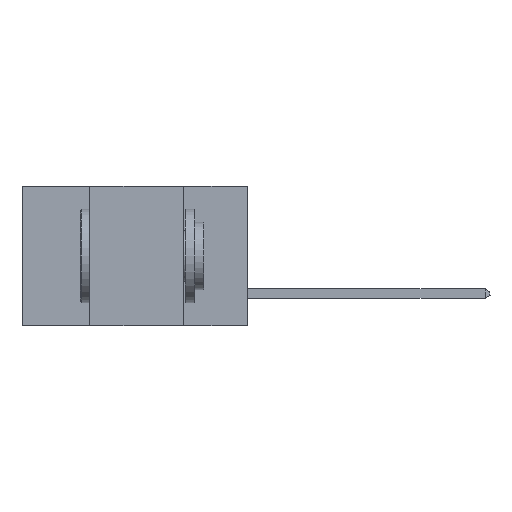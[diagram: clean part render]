
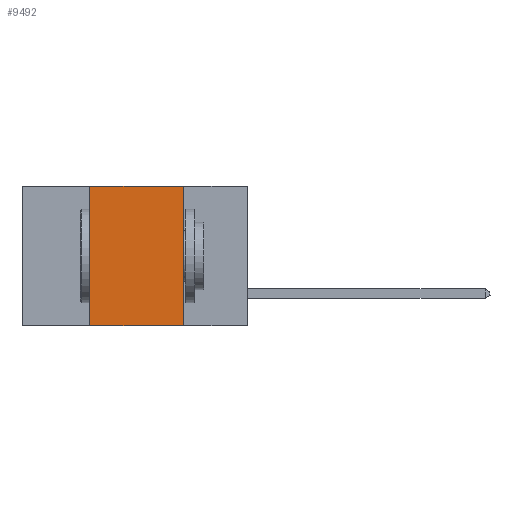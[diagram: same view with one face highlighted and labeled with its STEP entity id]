
A CAD part, left-side view. The second image highlights one B-rep face of the part: STEP entity #9492.
In plain terms, the highlighted planar face has unit normal (-1, 0, 0).
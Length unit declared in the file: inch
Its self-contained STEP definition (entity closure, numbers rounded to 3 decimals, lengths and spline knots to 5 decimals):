
#25 = AXIS2_PLACEMENT_3D ( 'NONE', #9663, #7342, #1075 ) ;
#957 = CARTESIAN_POINT ( 'NONE',  ( 0., 0.17, 0. ) ) ;
#1024 = DIRECTION ( 'NONE',  ( 0., 0., 1. ) ) ;
#1075 = DIRECTION ( 'NONE',  ( 0., 0., -1. ) ) ;
#1392 = ORIENTED_EDGE ( 'NONE', *, *, #3234, .F. ) ;
#1504 = CARTESIAN_POINT ( 'NONE',  ( 0., 0.17, 0. ) ) ;
#1588 = EDGE_CURVE ( 'NONE', #4769, #3531, #7890, .T. ) ;
#1631 = VECTOR ( 'NONE', #1024, 39.37008 ) ;
#1837 = EDGE_CURVE ( 'NONE', #5003, #3531, #3821, .T. ) ;
#1843 = VERTEX_POINT ( 'NONE', #9908 ) ;
#2128 = LINE ( 'NONE', #8068, #1631 ) ;
#2605 = ORIENTED_EDGE ( 'NONE', *, *, #1837, .F. ) ;
#3234 = EDGE_CURVE ( 'NONE', #4769, #1843, #2128, .T. ) ;
#3531 = VERTEX_POINT ( 'NONE', #6777 ) ;
#3821 = LINE ( 'NONE', #1504, #5123 ) ;
#3959 = ORIENTED_EDGE ( 'NONE', *, *, #9814, .F. ) ;
#4302 = PLANE ( 'NONE',  #25 ) ;
#4540 = FACE_OUTER_BOUND ( 'NONE', #5768, .T. ) ;
#4769 = VERTEX_POINT ( 'NONE', #7402 ) ;
#5003 = VERTEX_POINT ( 'NONE', #957 ) ;
#5123 = VECTOR ( 'NONE', #9191, 39.37008 ) ;
#5135 = LINE ( 'NONE', #5643, #6950 ) ;
#5643 = CARTESIAN_POINT ( 'NONE',  ( 0., 0.6, 0. ) ) ;
#5768 = EDGE_LOOP ( 'NONE', ( #2605, #3959, #1392, #7460 ) ) ;
#6777 = CARTESIAN_POINT ( 'NONE',  ( 0., 0.17, -0.37 ) ) ;
#6867 = DIRECTION ( 'NONE',  ( 0., -1., 0. ) ) ;
#6950 = VECTOR ( 'NONE', #8077, 39.37008 ) ;
#7342 = DIRECTION ( 'NONE',  ( 1., 0., 0. ) ) ;
#7402 = CARTESIAN_POINT ( 'NONE',  ( 0., 0.42, -0.37 ) ) ;
#7460 = ORIENTED_EDGE ( 'NONE', *, *, #1588, .T. ) ;
#7662 = VECTOR ( 'NONE', #6867, 39.37008 ) ;
#7890 = LINE ( 'NONE', #8431, #7662 ) ;
#8068 = CARTESIAN_POINT ( 'NONE',  ( 0., 0.42, 0. ) ) ;
#8077 = DIRECTION ( 'NONE',  ( 0., -1., 0. ) ) ;
#8431 = CARTESIAN_POINT ( 'NONE',  ( 0., 0.6, -0.37 ) ) ;
#9191 = DIRECTION ( 'NONE',  ( 0., 0., -1. ) ) ;
#9492 = ADVANCED_FACE ( 'NONE', ( #4540 ), #4302, .F. ) ;
#9663 = CARTESIAN_POINT ( 'NONE',  ( 0., 0.6, 0. ) ) ;
#9814 = EDGE_CURVE ( 'NONE', #1843, #5003, #5135, .T. ) ;
#9908 = CARTESIAN_POINT ( 'NONE',  ( 0., 0.42, 0. ) ) ;
